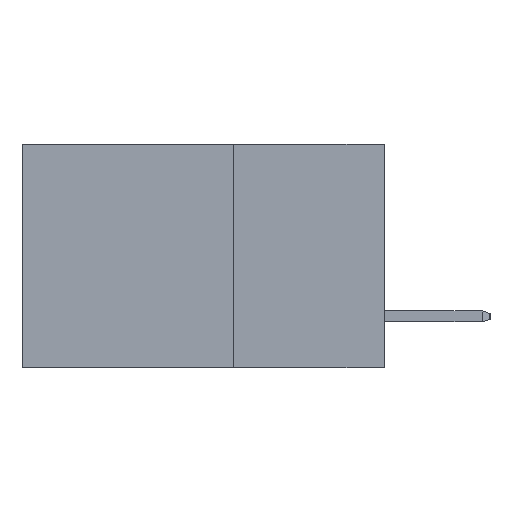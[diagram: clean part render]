
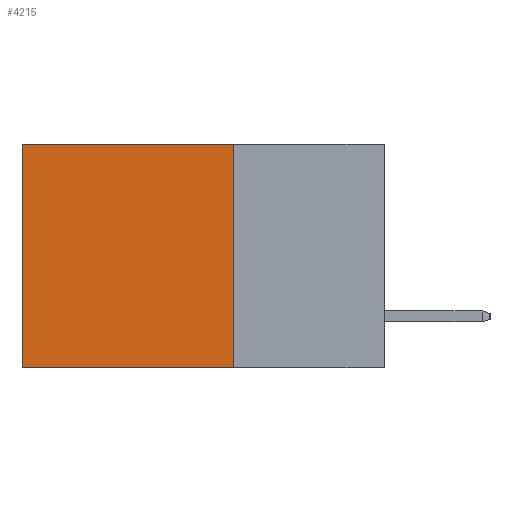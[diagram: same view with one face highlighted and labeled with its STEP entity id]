
A CAD part, left-side view. The second image highlights one B-rep face of the part: STEP entity #4215.
In plain terms, the highlighted planar face has unit normal (-1, 0, 0).
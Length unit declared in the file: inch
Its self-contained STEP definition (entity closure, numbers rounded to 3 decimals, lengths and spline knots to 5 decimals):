
#962 = PLANE ( 'NONE',  #16846 ) ;
#1595 = EDGE_CURVE ( 'NONE', #21470, #6246, #13199, .T. ) ;
#2071 = LINE ( 'NONE', #21994, #21661 ) ;
#2656 = EDGE_CURVE ( 'NONE', #21470, #22848, #9658, .T. ) ;
#2993 = VECTOR ( 'NONE', #22295, 39.37008 ) ;
#3099 = DIRECTION ( 'NONE',  ( 0., 0., -1. ) ) ;
#4100 = ORIENTED_EDGE ( 'NONE', *, *, #2656, .F. ) ;
#4215 = ADVANCED_FACE ( 'NONE', ( #4395 ), #962, .F. ) ;
#4395 = FACE_OUTER_BOUND ( 'NONE', #5735, .T. ) ;
#4477 = VECTOR ( 'NONE', #4856, 39.37008 ) ;
#4856 = DIRECTION ( 'NONE',  ( 0., 0., -1. ) ) ;
#5735 = EDGE_LOOP ( 'NONE', ( #13488, #16438, #4100, #5933 ) ) ;
#5933 = ORIENTED_EDGE ( 'NONE', *, *, #1595, .T. ) ;
#6246 = VERTEX_POINT ( 'NONE', #14224 ) ;
#7790 = CARTESIAN_POINT ( 'NONE',  ( 0.298, 0.6, -0.37 ) ) ;
#8276 = CARTESIAN_POINT ( 'NONE',  ( 0.298, 0.25, 0. ) ) ;
#9658 = LINE ( 'NONE', #22183, #4477 ) ;
#13199 = LINE ( 'NONE', #8276, #2993 ) ;
#13358 = EDGE_CURVE ( 'NONE', #22848, #23182, #15075, .T. ) ;
#13488 = ORIENTED_EDGE ( 'NONE', *, *, #16696, .T. ) ;
#14224 = CARTESIAN_POINT ( 'NONE',  ( 0.298, 0.6, 0. ) ) ;
#14423 = CARTESIAN_POINT ( 'NONE',  ( 0.298, 0.25, -0.37 ) ) ;
#14643 = CARTESIAN_POINT ( 'NONE',  ( 0.298, 0.25, 0. ) ) ;
#14832 = DIRECTION ( 'NONE',  ( 0., 1., 0. ) ) ;
#15075 = LINE ( 'NONE', #24095, #19468 ) ;
#16438 = ORIENTED_EDGE ( 'NONE', *, *, #13358, .F. ) ;
#16696 = EDGE_CURVE ( 'NONE', #6246, #23182, #2071, .T. ) ;
#16846 = AXIS2_PLACEMENT_3D ( 'NONE', #14643, #19790, #19761 ) ;
#19468 = VECTOR ( 'NONE', #14832, 39.37008 ) ;
#19761 = DIRECTION ( 'NONE',  ( 0., 0., -1. ) ) ;
#19790 = DIRECTION ( 'NONE',  ( 1., 0., 0. ) ) ;
#21470 = VERTEX_POINT ( 'NONE', #23220 ) ;
#21661 = VECTOR ( 'NONE', #3099, 39.37008 ) ;
#21994 = CARTESIAN_POINT ( 'NONE',  ( 0.298, 0.6, 0. ) ) ;
#22183 = CARTESIAN_POINT ( 'NONE',  ( 0.298, 0.25, 0. ) ) ;
#22295 = DIRECTION ( 'NONE',  ( 0., 1., 0. ) ) ;
#22848 = VERTEX_POINT ( 'NONE', #14423 ) ;
#23182 = VERTEX_POINT ( 'NONE', #7790 ) ;
#23220 = CARTESIAN_POINT ( 'NONE',  ( 0.298, 0.25, 0. ) ) ;
#24095 = CARTESIAN_POINT ( 'NONE',  ( 0.298, 0.25, -0.37 ) ) ;
